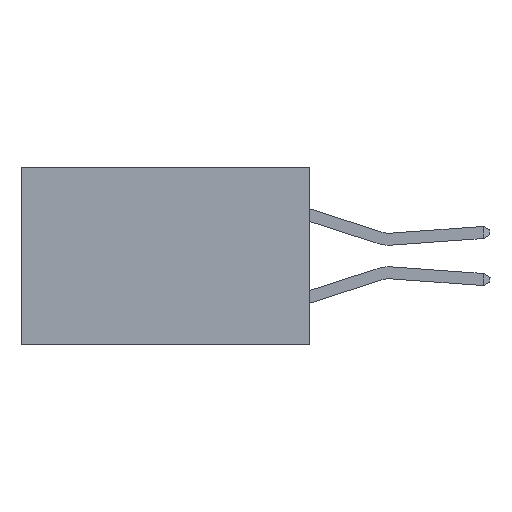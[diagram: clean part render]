
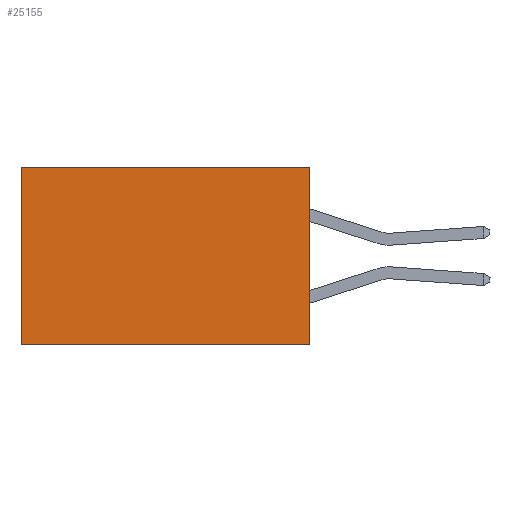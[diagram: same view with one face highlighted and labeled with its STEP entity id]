
A CAD part, left-side view. The second image highlights one B-rep face of the part: STEP entity #25155.
In plain terms, the highlighted planar face has unit normal (-1, 0, 0).
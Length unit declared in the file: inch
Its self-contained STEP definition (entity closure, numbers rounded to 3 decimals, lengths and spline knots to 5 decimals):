
#2321 = DIRECTION ( 'NONE',  ( 0., 1., 0. ) ) ;
#3791 = VERTEX_POINT ( 'NONE', #26162 ) ;
#4550 = CARTESIAN_POINT ( 'NONE',  ( 0.298, 0.6, 0. ) ) ;
#5841 = VECTOR ( 'NONE', #19266, 39.37008 ) ;
#6118 = VECTOR ( 'NONE', #2321, 39.37008 ) ;
#6207 = VECTOR ( 'NONE', #16760, 39.37008 ) ;
#6707 = DIRECTION ( 'NONE',  ( 0., 0., -1. ) ) ;
#6788 = CARTESIAN_POINT ( 'NONE',  ( 0.298, 0., 0. ) ) ;
#7487 = ORIENTED_EDGE ( 'NONE', *, *, #9710, .F. ) ;
#9700 = EDGE_CURVE ( 'NONE', #22707, #3791, #12000, .T. ) ;
#9710 = EDGE_CURVE ( 'NONE', #3791, #11591, #16464, .T. ) ;
#10312 = CARTESIAN_POINT ( 'NONE',  ( 0.298, 0., 0. ) ) ;
#11591 = VERTEX_POINT ( 'NONE', #19581 ) ;
#12000 = LINE ( 'NONE', #6788, #14758 ) ;
#14171 = EDGE_CURVE ( 'NONE', #28120, #11591, #19973, .T. ) ;
#14758 = VECTOR ( 'NONE', #27571, 39.37008 ) ;
#15384 = DIRECTION ( 'NONE',  ( 1., 0., 0. ) ) ;
#16464 = LINE ( 'NONE', #17695, #6118 ) ;
#16760 = DIRECTION ( 'NONE',  ( 0., 1., 0. ) ) ;
#17695 = CARTESIAN_POINT ( 'NONE',  ( 0.298, 0., -0.37 ) ) ;
#17801 = CARTESIAN_POINT ( 'NONE',  ( 0.298, 0., 0. ) ) ;
#18631 = ORIENTED_EDGE ( 'NONE', *, *, #18944, .T. ) ;
#18944 = EDGE_CURVE ( 'NONE', #22707, #28120, #27931, .T. ) ;
#19266 = DIRECTION ( 'NONE',  ( 0., 0., -1. ) ) ;
#19581 = CARTESIAN_POINT ( 'NONE',  ( 0.298, 0.6, -0.37 ) ) ;
#19973 = LINE ( 'NONE', #23771, #5841 ) ;
#21938 = PLANE ( 'NONE',  #26432 ) ;
#22707 = VERTEX_POINT ( 'NONE', #23086 ) ;
#23086 = CARTESIAN_POINT ( 'NONE',  ( 0.298, 0., 0. ) ) ;
#23166 = FACE_OUTER_BOUND ( 'NONE', #27426, .T. ) ;
#23771 = CARTESIAN_POINT ( 'NONE',  ( 0.298, 0.6, 0. ) ) ;
#24141 = ORIENTED_EDGE ( 'NONE', *, *, #9700, .F. ) ;
#25155 = ADVANCED_FACE ( 'NONE', ( #23166 ), #21938, .F. ) ;
#26039 = ORIENTED_EDGE ( 'NONE', *, *, #14171, .T. ) ;
#26162 = CARTESIAN_POINT ( 'NONE',  ( 0.298, 0., -0.37 ) ) ;
#26432 = AXIS2_PLACEMENT_3D ( 'NONE', #17801, #15384, #6707 ) ;
#27426 = EDGE_LOOP ( 'NONE', ( #26039, #7487, #24141, #18631 ) ) ;
#27571 = DIRECTION ( 'NONE',  ( 0., 0., -1. ) ) ;
#27931 = LINE ( 'NONE', #10312, #6207 ) ;
#28120 = VERTEX_POINT ( 'NONE', #4550 ) ;
